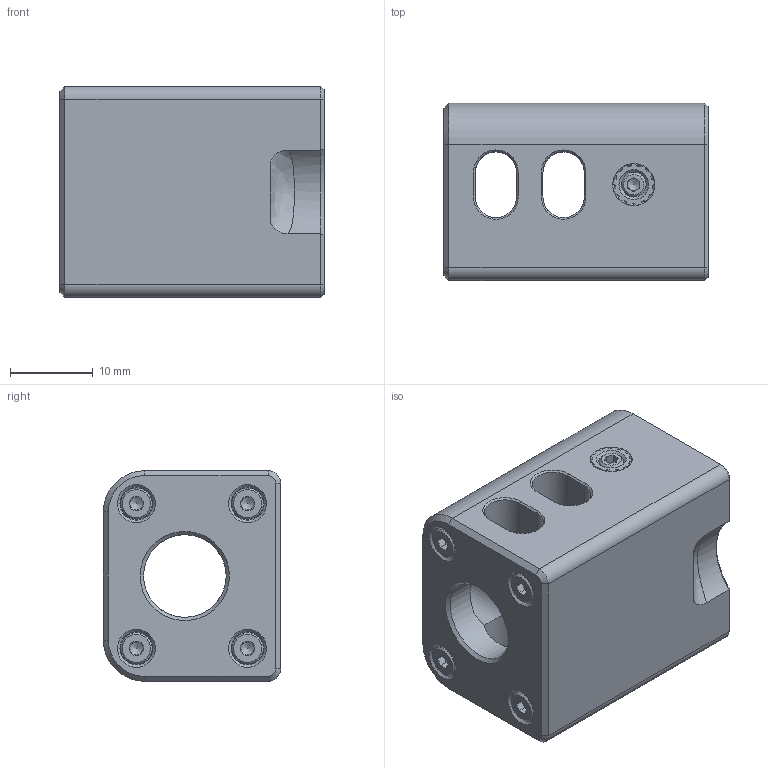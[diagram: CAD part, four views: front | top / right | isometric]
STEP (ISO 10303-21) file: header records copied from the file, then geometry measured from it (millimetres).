
FILE_DESCRIPTION(/* description */ (''),/* implementation_level */ '2;1');
FILE_NAME(/* name */ 'Glock Minor Comp.step',/* time_stamp */ '2023-03-25T01:16:58+13:00',/* author */ (''),/* organization */ (''),/* preprocessor_version */ 'ST-DEVELOPER v19.2',/* originating_system */ 'Autodesk Translation Framework v11.17.0.187',/* authorisation */ '');
FILE_SCHEMA (('AUTOMOTIVE_DESIGN { 1 0 10303 214 3 1 1 }'));
Length unit declared in the file: millimetre
Products named in the file (6): Cappin_JStark_Glock17_Gen3_Upper; Glock Minor Comp; VORON2.4_Assembly_M3 Threaded Insert; SBCP3-6 v2; M2_HEXNUT_LBNR2; M2x30_CSH-ST-M2-30_214
Assembly tree (13 placements, depth 3):
  Cappin_JStark_Glock17_Gen3_Upper
    Glock Minor Comp
      VORON2.4_Assembly_M3 Threaded Insert  x2
      SBCP3-6 v2  x2
    M2_HEXNUT_LBNR2  x4
    M2x30_CSH-ST-M2-30_214  x4
Bounding box: 32 x 21.46 x 25.53 mm (x, y, z)
Volume: 11915.8 mm3; surface area: 8172.8 mm2
Topology: 13 solids, 13 shells, 675 faces, 1730 edges, 1094 vertices
Faces by surface type: plane 226, bspline 173, cylinder 160, cone 111, torus 5
Full cylindrical faces by diameter (mm): 1.5 x2, 1.567 x4, 2 x4, 2.1 x4, 2.9 x2, 3 x2, 3.4 x2, 3.8 x4, 4 x4, 4.2 x2, 4.25 x2, 4.6 x2, 4.7 x2, 10 x1, 11.793 x4, 12.7 x4, 14.6 x1
Entity records: 17150 total; most frequent: CARTESIAN_POINT 7825, ORIENTED_EDGE 2138, DIRECTION 1527, EDGE_CURVE 1069, VERTEX_POINT 680, AXIS2_PLACEMENT_3D 569, EDGE_LOOP 443, B_SPLINE_CURVE_WITH_KNOTS 417
